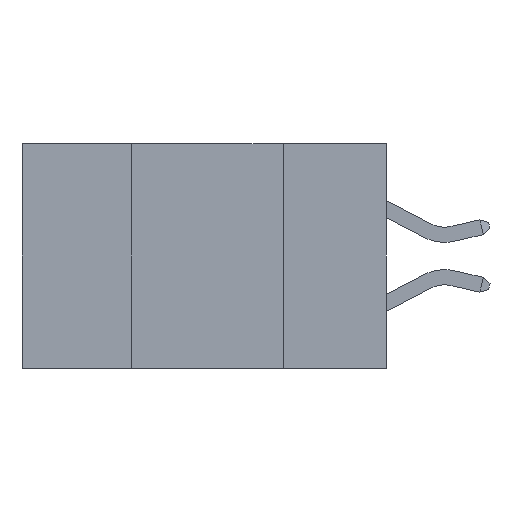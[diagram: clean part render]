
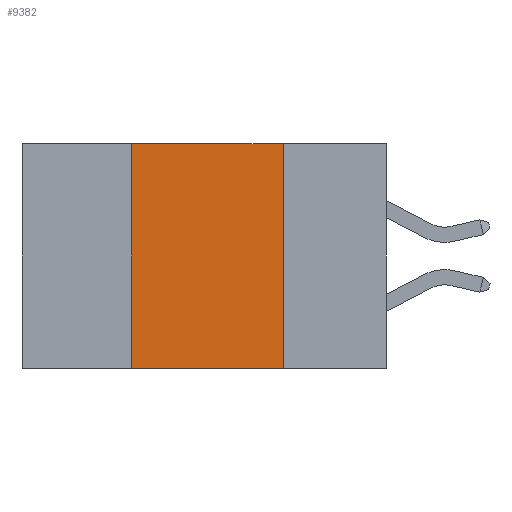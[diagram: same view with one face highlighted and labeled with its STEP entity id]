
A CAD part, left-side view. The second image highlights one B-rep face of the part: STEP entity #9382.
In plain terms, the highlighted planar face has unit normal (-1, 0, 0).
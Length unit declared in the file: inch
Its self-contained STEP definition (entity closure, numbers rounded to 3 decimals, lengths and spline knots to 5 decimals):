
#218 = LINE ( 'NONE', #8956, #9818 ) ;
#229 = DIRECTION ( 'NONE',  ( 0., 0., -1. ) ) ;
#371 = VERTEX_POINT ( 'NONE', #11697 ) ;
#547 = VERTEX_POINT ( 'NONE', #10072 ) ;
#615 = EDGE_CURVE ( 'NONE', #8107, #9745, #218, .T. ) ;
#881 = LINE ( 'NONE', #10987, #10495 ) ;
#997 = DIRECTION ( 'NONE',  ( 0., 0., -1. ) ) ;
#1003 = EDGE_LOOP ( 'NONE', ( #4645, #11445, #6479, #10141 ) ) ;
#1886 = EDGE_CURVE ( 'NONE', #8107, #371, #881, .T. ) ;
#3004 = PLANE ( 'NONE',  #4884 ) ;
#3130 = VECTOR ( 'NONE', #11261, 39.37008 ) ;
#3794 = CARTESIAN_POINT ( 'NONE',  ( 0., 0.17, -0.37 ) ) ;
#3860 = CARTESIAN_POINT ( 'NONE',  ( 0., 0.6, 0. ) ) ;
#4645 = ORIENTED_EDGE ( 'NONE', *, *, #7344, .F. ) ;
#4884 = AXIS2_PLACEMENT_3D ( 'NONE', #11321, #5843, #229 ) ;
#5628 = LINE ( 'NONE', #3860, #3130 ) ;
#5658 = EDGE_CURVE ( 'NONE', #371, #547, #5628, .T. ) ;
#5843 = DIRECTION ( 'NONE',  ( 1., 0., 0. ) ) ;
#6313 = CARTESIAN_POINT ( 'NONE',  ( 0., 0.17, -0.37 ) ) ;
#6479 = ORIENTED_EDGE ( 'NONE', *, *, #1886, .F. ) ;
#6782 = CARTESIAN_POINT ( 'NONE',  ( 0., 0.42, -0.37 ) ) ;
#7344 = EDGE_CURVE ( 'NONE', #547, #9745, #10400, .T. ) ;
#8107 = VERTEX_POINT ( 'NONE', #6782 ) ;
#8656 = FACE_OUTER_BOUND ( 'NONE', #1003, .T. ) ;
#8956 = CARTESIAN_POINT ( 'NONE',  ( 0., 0.6, -0.37 ) ) ;
#9274 = DIRECTION ( 'NONE',  ( 0., -1., 0. ) ) ;
#9382 = ADVANCED_FACE ( 'NONE', ( #8656 ), #3004, .F. ) ;
#9658 = VECTOR ( 'NONE', #997, 39.37008 ) ;
#9745 = VERTEX_POINT ( 'NONE', #6313 ) ;
#9818 = VECTOR ( 'NONE', #9274, 39.37008 ) ;
#10072 = CARTESIAN_POINT ( 'NONE',  ( 0., 0.17, 0. ) ) ;
#10141 = ORIENTED_EDGE ( 'NONE', *, *, #615, .T. ) ;
#10400 = LINE ( 'NONE', #3794, #9658 ) ;
#10495 = VECTOR ( 'NONE', #11521, 39.37008 ) ;
#10987 = CARTESIAN_POINT ( 'NONE',  ( 0., 0.42, -0.37 ) ) ;
#11261 = DIRECTION ( 'NONE',  ( 0., -1., 0. ) ) ;
#11321 = CARTESIAN_POINT ( 'NONE',  ( 0., 0.6, 0. ) ) ;
#11445 = ORIENTED_EDGE ( 'NONE', *, *, #5658, .F. ) ;
#11521 = DIRECTION ( 'NONE',  ( 0., 0., 1. ) ) ;
#11697 = CARTESIAN_POINT ( 'NONE',  ( 0., 0.42, 0. ) ) ;
